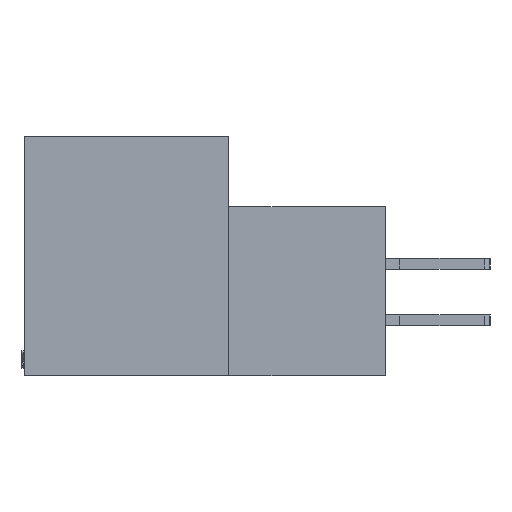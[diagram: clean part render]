
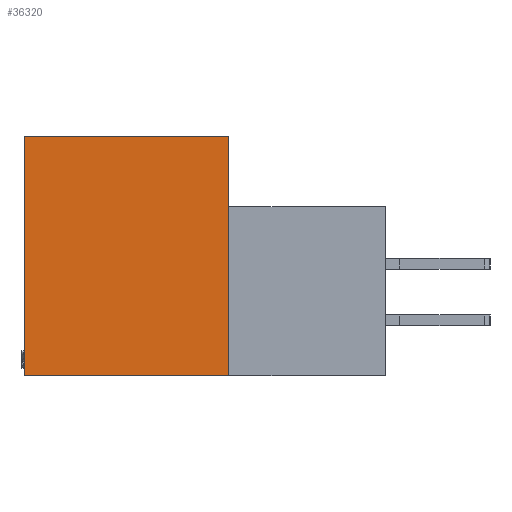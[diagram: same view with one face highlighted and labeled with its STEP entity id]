
A CAD part, left-side view. The second image highlights one B-rep face of the part: STEP entity #36320.
In plain terms, the highlighted planar face has unit normal (-1, 0, 0).
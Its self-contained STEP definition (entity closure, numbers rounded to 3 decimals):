
#368 = CARTESIAN_POINT ( 'NONE',  ( 0., 11.506, -13.487 ) ) ;
#2571 = LINE ( 'NONE', #21442, #42317 ) ;
#3940 = ORIENTED_EDGE ( 'NONE', *, *, #22687, .F. ) ;
#4324 = DIRECTION ( 'NONE',  ( 0., 0., -1. ) ) ;
#4518 = VERTEX_POINT ( 'NONE', #25376 ) ;
#6896 = VECTOR ( 'NONE', #17588, 1000. ) ;
#8694 = EDGE_CURVE ( 'NONE', #4518, #18497, #27239, .T. ) ;
#9687 = FACE_OUTER_BOUND ( 'NONE', #44553, .T. ) ;
#11235 = CARTESIAN_POINT ( 'NONE',  ( 0., 0., 0. ) ) ;
#11282 = PLANE ( 'NONE',  #12588 ) ;
#11578 = CARTESIAN_POINT ( 'NONE',  ( 0., 0., 0. ) ) ;
#12588 = AXIS2_PLACEMENT_3D ( 'NONE', #39657, #43022, #4324 ) ;
#12598 = CARTESIAN_POINT ( 'NONE',  ( 0., 11.506, 0. ) ) ;
#13880 = ORIENTED_EDGE ( 'NONE', *, *, #42316, .F. ) ;
#16147 = CARTESIAN_POINT ( 'NONE',  ( 0., 11.506, 0. ) ) ;
#17588 = DIRECTION ( 'NONE',  ( 0., 1., 0. ) ) ;
#18497 = VERTEX_POINT ( 'NONE', #368 ) ;
#18779 = DIRECTION ( 'NONE',  ( 0., 0., -1. ) ) ;
#20875 = VERTEX_POINT ( 'NONE', #11235 ) ;
#21442 = CARTESIAN_POINT ( 'NONE',  ( 0., 11.506, -13.487 ) ) ;
#22687 = EDGE_CURVE ( 'NONE', #32883, #20875, #38127, .T. ) ;
#23338 = DIRECTION ( 'NONE',  ( 0., -1., 0. ) ) ;
#24726 = LINE ( 'NONE', #11578, #31898 ) ;
#25376 = CARTESIAN_POINT ( 'NONE',  ( 0., 0., -13.487 ) ) ;
#27239 = LINE ( 'NONE', #38871, #6896 ) ;
#28836 = EDGE_CURVE ( 'NONE', #20875, #4518, #24726, .T. ) ;
#31753 = DIRECTION ( 'NONE',  ( 0., 0., 1. ) ) ;
#31898 = VECTOR ( 'NONE', #18779, 1000. ) ;
#32105 = ORIENTED_EDGE ( 'NONE', *, *, #28836, .F. ) ;
#32883 = VERTEX_POINT ( 'NONE', #16147 ) ;
#33102 = VECTOR ( 'NONE', #23338, 1000. ) ;
#36320 = ADVANCED_FACE ( 'NONE', ( #9687 ), #11282, .F. ) ;
#38127 = LINE ( 'NONE', #12598, #33102 ) ;
#38871 = CARTESIAN_POINT ( 'NONE',  ( 0., -8.814, -13.487 ) ) ;
#39657 = CARTESIAN_POINT ( 'NONE',  ( 0., 0., 0. ) ) ;
#41017 = ORIENTED_EDGE ( 'NONE', *, *, #8694, .F. ) ;
#42316 = EDGE_CURVE ( 'NONE', #18497, #32883, #2571, .T. ) ;
#42317 = VECTOR ( 'NONE', #31753, 1000. ) ;
#43022 = DIRECTION ( 'NONE',  ( 1., 0., 0. ) ) ;
#44553 = EDGE_LOOP ( 'NONE', ( #41017, #32105, #3940, #13880 ) ) ;
